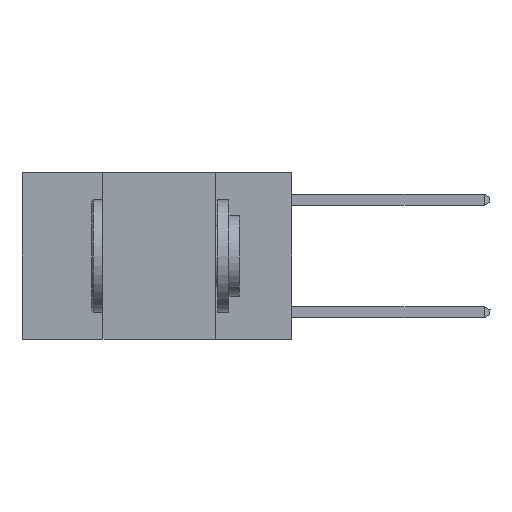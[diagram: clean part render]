
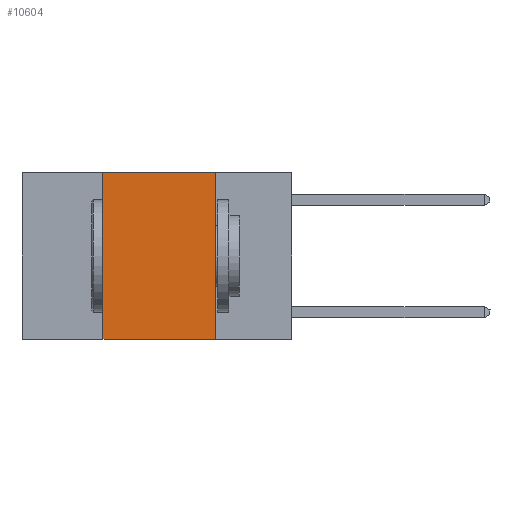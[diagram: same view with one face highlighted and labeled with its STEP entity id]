
A CAD part, left-side view. The second image highlights one B-rep face of the part: STEP entity #10604.
In plain terms, the highlighted planar face has unit normal (-1, 0, 0).
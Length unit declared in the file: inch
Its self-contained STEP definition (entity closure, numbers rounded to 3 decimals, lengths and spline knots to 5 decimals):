
#517 = VERTEX_POINT ( 'NONE', #3939 ) ;
#588 = DIRECTION ( 'NONE',  ( 0., -1., 0. ) ) ;
#616 = LINE ( 'NONE', #6767, #11960 ) ;
#691 = CARTESIAN_POINT ( 'NONE',  ( 0., 0.6, -0.37 ) ) ;
#1362 = EDGE_CURVE ( 'NONE', #6271, #12587, #12849, .T. ) ;
#1887 = CARTESIAN_POINT ( 'NONE',  ( 0., 0.6, 0. ) ) ;
#2231 = LINE ( 'NONE', #3755, #10052 ) ;
#2913 = CARTESIAN_POINT ( 'NONE',  ( 0., 0.17, -0.37 ) ) ;
#3113 = EDGE_CURVE ( 'NONE', #6271, #517, #616, .T. ) ;
#3190 = CARTESIAN_POINT ( 'NONE',  ( 0., 0.17, 0. ) ) ;
#3277 = VECTOR ( 'NONE', #7463, 39.37008 ) ;
#3614 = LINE ( 'NONE', #1887, #3277 ) ;
#3755 = CARTESIAN_POINT ( 'NONE',  ( 0., 0.17, 0. ) ) ;
#3939 = CARTESIAN_POINT ( 'NONE',  ( 0., 0.42, 0. ) ) ;
#4890 = DIRECTION ( 'NONE',  ( 0., 0., -1. ) ) ;
#5447 = PLANE ( 'NONE',  #6086 ) ;
#5848 = CARTESIAN_POINT ( 'NONE',  ( 0., 0.42, -0.37 ) ) ;
#5934 = EDGE_CURVE ( 'NONE', #12769, #12587, #2231, .T. ) ;
#6086 = AXIS2_PLACEMENT_3D ( 'NONE', #13093, #6586, #14193 ) ;
#6271 = VERTEX_POINT ( 'NONE', #5848 ) ;
#6553 = DIRECTION ( 'NONE',  ( 0., 0., 1. ) ) ;
#6586 = DIRECTION ( 'NONE',  ( 1., 0., 0. ) ) ;
#6767 = CARTESIAN_POINT ( 'NONE',  ( 0., 0.42, 0. ) ) ;
#7119 = ORIENTED_EDGE ( 'NONE', *, *, #5934, .F. ) ;
#7158 = ORIENTED_EDGE ( 'NONE', *, *, #10482, .F. ) ;
#7234 = ORIENTED_EDGE ( 'NONE', *, *, #3113, .F. ) ;
#7248 = ORIENTED_EDGE ( 'NONE', *, *, #1362, .T. ) ;
#7463 = DIRECTION ( 'NONE',  ( 0., -1., 0. ) ) ;
#10052 = VECTOR ( 'NONE', #4890, 39.37008 ) ;
#10401 = FACE_OUTER_BOUND ( 'NONE', #10911, .T. ) ;
#10482 = EDGE_CURVE ( 'NONE', #517, #12769, #3614, .T. ) ;
#10604 = ADVANCED_FACE ( 'NONE', ( #10401 ), #5447, .F. ) ;
#10911 = EDGE_LOOP ( 'NONE', ( #7119, #7158, #7234, #7248 ) ) ;
#11960 = VECTOR ( 'NONE', #6553, 39.37008 ) ;
#12496 = VECTOR ( 'NONE', #588, 39.37008 ) ;
#12587 = VERTEX_POINT ( 'NONE', #2913 ) ;
#12769 = VERTEX_POINT ( 'NONE', #3190 ) ;
#12849 = LINE ( 'NONE', #691, #12496 ) ;
#13093 = CARTESIAN_POINT ( 'NONE',  ( 0., 0.6, 0. ) ) ;
#14193 = DIRECTION ( 'NONE',  ( 0., 0., -1. ) ) ;
